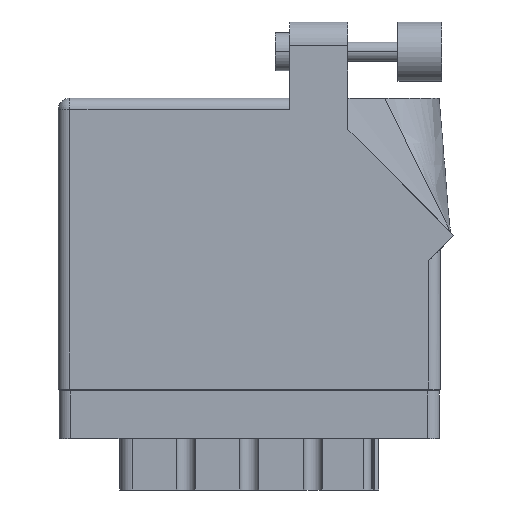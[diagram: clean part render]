
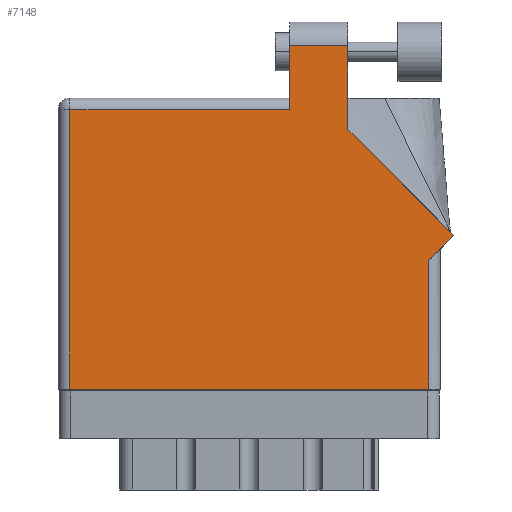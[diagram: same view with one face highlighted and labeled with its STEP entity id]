
A CAD part, front view. The second image highlights one B-rep face of the part: STEP entity #7148.
In plain terms, the highlighted face is planar.
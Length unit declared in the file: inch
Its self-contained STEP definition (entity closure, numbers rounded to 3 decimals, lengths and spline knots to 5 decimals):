
#1997 = VERTEX_POINT ( 'NONE', #18636 ) ;
#2140 = CARTESIAN_POINT ( 'NONE',  ( 1.948, 0., 0. ) ) ;
#2415 = VECTOR ( 'NONE', #27391, 39.37008 ) ;
#2934 = CARTESIAN_POINT ( 'NONE',  ( 0., 0., 0. ) ) ;
#4973 = VERTEX_POINT ( 'NONE', #5325 ) ;
#5257 = CARTESIAN_POINT ( 'NONE',  ( 1.948, 0.737, 0. ) ) ;
#5307 = ORIENTED_EDGE ( 'NONE', *, *, #33693, .T. ) ;
#5325 = CARTESIAN_POINT ( 'NONE',  ( 1.217, 1.468, 0. ) ) ;
#5442 = VECTOR ( 'NONE', #31353, 39.37008 ) ;
#5782 = VECTOR ( 'NONE', #16307, 39.37008 ) ;
#6377 = DIRECTION ( 'NONE',  ( 0., 1., 0. ) ) ;
#7055 = LINE ( 'NONE', #25087, #26424 ) ;
#7148 = ADVANCED_FACE ( 'NONE', ( #35640 ), #24342, .F. ) ;
#7335 = CARTESIAN_POINT ( 'NONE',  ( 0., 1.468, 0. ) ) ;
#7838 = CARTESIAN_POINT ( 'NONE',  ( 1.217, 1.53, 0. ) ) ;
#8205 = CARTESIAN_POINT ( 'NONE',  ( 0.062, 1.468, 0. ) ) ;
#8657 = CARTESIAN_POINT ( 'NONE',  ( 1.524, 1.36442, 0. ) ) ;
#9188 = CARTESIAN_POINT ( 'NONE',  ( 1.524, 1.36442, 0. ) ) ;
#10267 = AXIS2_PLACEMENT_3D ( 'NONE', #35995, #27150, #12487 ) ;
#10694 = VERTEX_POINT ( 'NONE', #26136 ) ;
#11800 = EDGE_CURVE ( 'NONE', #4973, #13861, #21625, .T. ) ;
#12487 = DIRECTION ( 'NONE',  ( -1., 0., 0. ) ) ;
#12889 = VECTOR ( 'NONE', #28197, 39.37008 ) ;
#13249 = LINE ( 'NONE', #27555, #15922 ) ;
#13443 = VERTEX_POINT ( 'NONE', #22149 ) ;
#13674 = LINE ( 'NONE', #31007, #5782 ) ;
#13751 = EDGE_LOOP ( 'NONE', ( #32027, #15653, #14588, #35499, #29211, #13993, #5307, #21225, #31351 ) ) ;
#13861 = VERTEX_POINT ( 'NONE', #8205 ) ;
#13993 = ORIENTED_EDGE ( 'NONE', *, *, #27775, .T. ) ;
#14553 = VERTEX_POINT ( 'NONE', #35126 ) ;
#14588 = ORIENTED_EDGE ( 'NONE', *, *, #20770, .T. ) ;
#15653 = ORIENTED_EDGE ( 'NONE', *, *, #29327, .T. ) ;
#15922 = VECTOR ( 'NONE', #22274, 39.37008 ) ;
#15937 = EDGE_CURVE ( 'NONE', #13861, #14553, #36783, .T. ) ;
#16307 = DIRECTION ( 'NONE',  ( -0.707, 0.707, 0. ) ) ;
#16675 = LINE ( 'NONE', #7838, #5442 ) ;
#16948 = VERTEX_POINT ( 'NONE', #8657 ) ;
#18636 = CARTESIAN_POINT ( 'NONE',  ( 1.948, 0.675, 0. ) ) ;
#18811 = DIRECTION ( 'NONE',  ( -1., 0., 0. ) ) ;
#19066 = DIRECTION ( 'NONE',  ( 0.707, 0.707, 0. ) ) ;
#19894 = VECTOR ( 'NONE', #18811, 39.37008 ) ;
#20060 = DIRECTION ( 'NONE',  ( 1., 0., 0. ) ) ;
#20770 = EDGE_CURVE ( 'NONE', #10694, #4973, #16675, .T. ) ;
#21225 = ORIENTED_EDGE ( 'NONE', *, *, #31402, .T. ) ;
#21409 = LINE ( 'NONE', #9188, #35666 ) ;
#21625 = LINE ( 'NONE', #7335, #19894 ) ;
#22149 = CARTESIAN_POINT ( 'NONE',  ( 2.08071, 0.80771, 0. ) ) ;
#22274 = DIRECTION ( 'NONE',  ( -1., 0., 0. ) ) ;
#23709 = EDGE_CURVE ( 'NONE', #16948, #29256, #21409, .T. ) ;
#24306 = VECTOR ( 'NONE', #20060, 39.37008 ) ;
#24342 = PLANE ( 'NONE',  #10267 ) ;
#24548 = CARTESIAN_POINT ( 'NONE',  ( 1.524, 1.805, 0. ) ) ;
#25087 = CARTESIAN_POINT ( 'NONE',  ( 2.01, 0.737, 0. ) ) ;
#26136 = CARTESIAN_POINT ( 'NONE',  ( 1.217, 1.805, 0. ) ) ;
#26424 = VECTOR ( 'NONE', #19066, 39.37008 ) ;
#27150 = DIRECTION ( 'NONE',  ( 0., 0., -1. ) ) ;
#27391 = DIRECTION ( 'NONE',  ( 0., -1., 0. ) ) ;
#27555 = CARTESIAN_POINT ( 'NONE',  ( 1.217, 1.805, 0. ) ) ;
#27775 = EDGE_CURVE ( 'NONE', #14553, #35443, #28539, .T. ) ;
#28197 = DIRECTION ( 'NONE',  ( 0., 1., 0. ) ) ;
#28539 = LINE ( 'NONE', #2934, #24306 ) ;
#29211 = ORIENTED_EDGE ( 'NONE', *, *, #15937, .T. ) ;
#29256 = VERTEX_POINT ( 'NONE', #24548 ) ;
#29327 = EDGE_CURVE ( 'NONE', #29256, #10694, #13249, .T. ) ;
#30232 = EDGE_CURVE ( 'NONE', #13443, #16948, #13674, .T. ) ;
#31007 = CARTESIAN_POINT ( 'NONE',  ( 2.08071, 0.80771, 0. ) ) ;
#31351 = ORIENTED_EDGE ( 'NONE', *, *, #30232, .T. ) ;
#31353 = DIRECTION ( 'NONE',  ( 0., -1., 0. ) ) ;
#31402 = EDGE_CURVE ( 'NONE', #1997, #13443, #7055, .T. ) ;
#32027 = ORIENTED_EDGE ( 'NONE', *, *, #23709, .T. ) ;
#33693 = EDGE_CURVE ( 'NONE', #35443, #1997, #34420, .T. ) ;
#33969 = CARTESIAN_POINT ( 'NONE',  ( 0.062, 0., 0. ) ) ;
#34420 = LINE ( 'NONE', #5257, #12889 ) ;
#35126 = CARTESIAN_POINT ( 'NONE',  ( 0.062, 0., 0. ) ) ;
#35443 = VERTEX_POINT ( 'NONE', #2140 ) ;
#35499 = ORIENTED_EDGE ( 'NONE', *, *, #11800, .T. ) ;
#35640 = FACE_OUTER_BOUND ( 'NONE', #13751, .T. ) ;
#35666 = VECTOR ( 'NONE', #6377, 39.37008 ) ;
#35995 = CARTESIAN_POINT ( 'NONE',  ( 0., 1.53, 0. ) ) ;
#36783 = LINE ( 'NONE', #33969, #2415 ) ;
